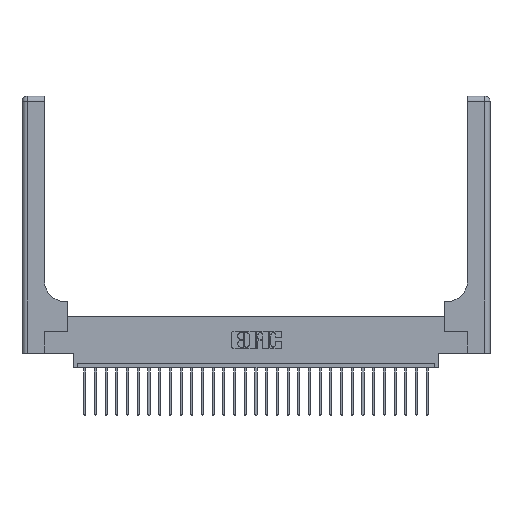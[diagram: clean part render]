
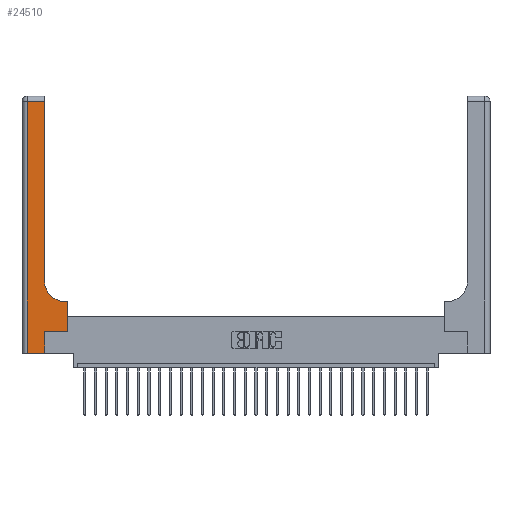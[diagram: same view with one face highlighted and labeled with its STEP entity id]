
A CAD part, top view. The second image highlights one B-rep face of the part: STEP entity #24510.
In plain terms, the highlighted planar face has unit normal (0, 0, 1).
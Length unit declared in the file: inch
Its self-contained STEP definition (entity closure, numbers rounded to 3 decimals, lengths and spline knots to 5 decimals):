
#131 = CARTESIAN_POINT ( 'NONE',  ( 0., 0., 0.37 ) ) ;
#403 = DIRECTION ( 'NONE',  ( 1., 0., 0. ) ) ;
#710 = DIRECTION ( 'NONE',  ( 0., 1., 0. ) ) ;
#1421 = DIRECTION ( 'NONE',  ( -1., 0., 0. ) ) ;
#1437 = VECTOR ( 'NONE', #1421, 39.37008 ) ;
#1827 = EDGE_CURVE ( 'NONE', #19913, #10586, #9132, .T. ) ;
#1888 = LINE ( 'NONE', #21517, #24754 ) ;
#2218 = LINE ( 'NONE', #13393, #8724 ) ;
#2820 = VECTOR ( 'NONE', #18384, 39.37008 ) ;
#3267 = EDGE_CURVE ( 'NONE', #10586, #19468, #1888, .T. ) ;
#3441 = ORIENTED_EDGE ( 'NONE', *, *, #1827, .T. ) ;
#3754 = EDGE_CURVE ( 'NONE', #19468, #7643, #2218, .T. ) ;
#4083 = EDGE_CURVE ( 'NONE', #16731, #26277, #24377, .T. ) ;
#4185 = EDGE_CURVE ( 'NONE', #20720, #26234, #14888, .T. ) ;
#4252 = DIRECTION ( 'NONE',  ( -1., 0., 0. ) ) ;
#4290 = CARTESIAN_POINT ( 'NONE',  ( 0.51, 0.6, 0.37 ) ) ;
#5453 = LINE ( 'NONE', #10810, #16235 ) ;
#5678 = VERTEX_POINT ( 'NONE', #22148 ) ;
#5928 = CARTESIAN_POINT ( 'NONE',  ( 0.26, 2.94, 0.37 ) ) ;
#6778 = ORIENTED_EDGE ( 'NONE', *, *, #12263, .T. ) ;
#7643 = VERTEX_POINT ( 'NONE', #20504 ) ;
#7812 = CARTESIAN_POINT ( 'NONE',  ( 0.26, 3., 0.37 ) ) ;
#7845 = AXIS2_PLACEMENT_3D ( 'NONE', #16593, #8129, #24820 ) ;
#8034 = LINE ( 'NONE', #7812, #2820 ) ;
#8071 = CARTESIAN_POINT ( 'NONE',  ( 0.06, 2.94, 0.37 ) ) ;
#8129 = DIRECTION ( 'NONE',  ( 0., 0., -1. ) ) ;
#8294 = ORIENTED_EDGE ( 'NONE', *, *, #21311, .T. ) ;
#8724 = VECTOR ( 'NONE', #25678, 39.37008 ) ;
#8736 = DIRECTION ( 'NONE',  ( 0., 0., -1. ) ) ;
#8812 = DIRECTION ( 'NONE',  ( 0., 1., 0. ) ) ;
#8947 = ORIENTED_EDGE ( 'NONE', *, *, #4185, .T. ) ;
#9132 = LINE ( 'NONE', #131, #9763 ) ;
#9763 = VECTOR ( 'NONE', #403, 39.37008 ) ;
#9942 = AXIS2_PLACEMENT_3D ( 'NONE', #21255, #8736, #15026 ) ;
#10586 = VERTEX_POINT ( 'NONE', #22510 ) ;
#10810 = CARTESIAN_POINT ( 'NONE',  ( 0.528, 0.25, 0.37 ) ) ;
#12263 = EDGE_CURVE ( 'NONE', #5678, #20720, #23007, .T. ) ;
#12870 = ORIENTED_EDGE ( 'NONE', *, *, #3267, .T. ) ;
#13393 = CARTESIAN_POINT ( 'NONE',  ( 0.265, 0.25, 0.37 ) ) ;
#13588 = ORIENTED_EDGE ( 'NONE', *, *, #26199, .T. ) ;
#13651 = FACE_OUTER_BOUND ( 'NONE', #17143, .T. ) ;
#13901 = CARTESIAN_POINT ( 'NONE',  ( 0.26, 0.6, 0.37 ) ) ;
#14888 = CIRCLE ( 'NONE', #7845, 0.25 ) ;
#15009 = CARTESIAN_POINT ( 'NONE',  ( 0.06, 3., 0.37 ) ) ;
#15026 = DIRECTION ( 'NONE',  ( -1., 0., 0. ) ) ;
#15088 = ORIENTED_EDGE ( 'NONE', *, *, #4083, .T. ) ;
#15206 = ORIENTED_EDGE ( 'NONE', *, *, #17563, .T. ) ;
#15992 = CARTESIAN_POINT ( 'NONE',  ( 0.06, 0., 0.37 ) ) ;
#16053 = VECTOR ( 'NONE', #23145, 39.37008 ) ;
#16235 = VECTOR ( 'NONE', #8812, 39.37008 ) ;
#16593 = CARTESIAN_POINT ( 'NONE',  ( 0.51, 0.85, 0.37 ) ) ;
#16731 = VERTEX_POINT ( 'NONE', #5928 ) ;
#16853 = VECTOR ( 'NONE', #4252, 39.37008 ) ;
#17143 = EDGE_LOOP ( 'NONE', ( #13588, #15088, #8294, #3441, #12870, #19655, #15206, #6778, #8947 ) ) ;
#17563 = EDGE_CURVE ( 'NONE', #7643, #5678, #5453, .T. ) ;
#18384 = DIRECTION ( 'NONE',  ( 0., 1., 0. ) ) ;
#18692 = CARTESIAN_POINT ( 'NONE',  ( 0., 2.94, 0.37 ) ) ;
#19175 = PLANE ( 'NONE',  #9942 ) ;
#19468 = VERTEX_POINT ( 'NONE', #26970 ) ;
#19655 = ORIENTED_EDGE ( 'NONE', *, *, #3754, .T. ) ;
#19913 = VERTEX_POINT ( 'NONE', #15992 ) ;
#20504 = CARTESIAN_POINT ( 'NONE',  ( 0.528, 0.25, 0.37 ) ) ;
#20720 = VERTEX_POINT ( 'NONE', #4290 ) ;
#21255 = CARTESIAN_POINT ( 'NONE',  ( 0., 3., 0.37 ) ) ;
#21311 = EDGE_CURVE ( 'NONE', #26277, #19913, #26834, .T. ) ;
#21517 = CARTESIAN_POINT ( 'NONE',  ( 0.265, 0., 0.37 ) ) ;
#22148 = CARTESIAN_POINT ( 'NONE',  ( 0.528, 0.6, 0.37 ) ) ;
#22510 = CARTESIAN_POINT ( 'NONE',  ( 0.265, 0., 0.37 ) ) ;
#23007 = LINE ( 'NONE', #13901, #1437 ) ;
#23145 = DIRECTION ( 'NONE',  ( 0., -1., 0. ) ) ;
#24377 = LINE ( 'NONE', #18692, #16853 ) ;
#24510 = ADVANCED_FACE ( 'NONE', ( #13651 ), #19175, .F. ) ;
#24754 = VECTOR ( 'NONE', #710, 39.37008 ) ;
#24820 = DIRECTION ( 'NONE',  ( 1., 0., 0. ) ) ;
#25678 = DIRECTION ( 'NONE',  ( 1., 0., 0. ) ) ;
#26199 = EDGE_CURVE ( 'NONE', #26234, #16731, #8034, .T. ) ;
#26234 = VERTEX_POINT ( 'NONE', #26683 ) ;
#26277 = VERTEX_POINT ( 'NONE', #8071 ) ;
#26683 = CARTESIAN_POINT ( 'NONE',  ( 0.26, 0.85, 0.37 ) ) ;
#26834 = LINE ( 'NONE', #15009, #16053 ) ;
#26970 = CARTESIAN_POINT ( 'NONE',  ( 0.265, 0.25, 0.37 ) ) ;
